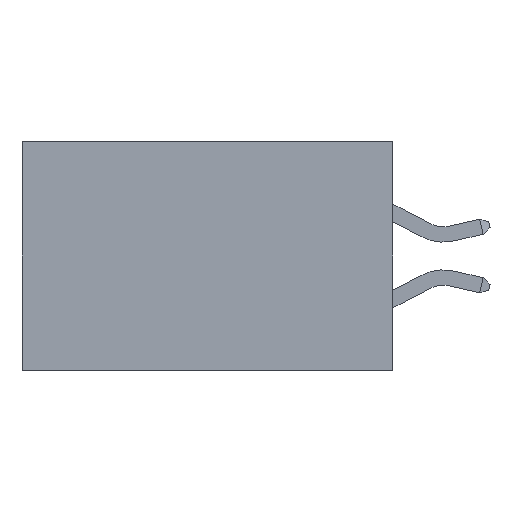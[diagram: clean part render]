
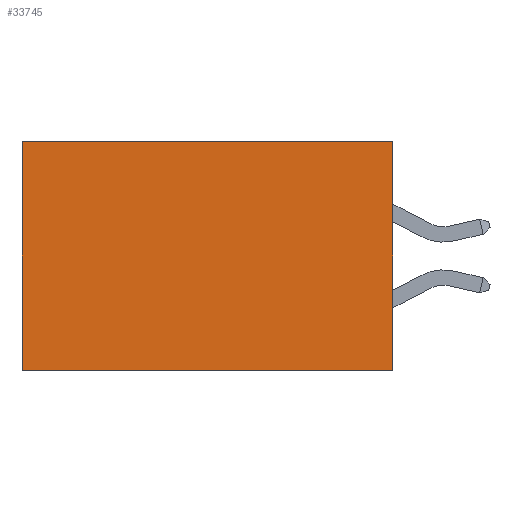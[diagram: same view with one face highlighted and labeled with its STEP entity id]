
A CAD part, left-side view. The second image highlights one B-rep face of the part: STEP entity #33745.
In plain terms, the highlighted planar face has unit normal (-1, 0, 0).
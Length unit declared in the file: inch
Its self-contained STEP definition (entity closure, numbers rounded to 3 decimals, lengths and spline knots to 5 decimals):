
#3464 = CARTESIAN_POINT ( 'NONE',  ( 0.2875, 0., 0. ) ) ;
#3906 = EDGE_CURVE ( 'NONE', #8949, #22092, #23940, .T. ) ;
#4215 = AXIS2_PLACEMENT_3D ( 'NONE', #3464, #6628, #9650 ) ;
#6011 = CARTESIAN_POINT ( 'NONE',  ( 0.2875, 0.6, 0. ) ) ;
#6628 = DIRECTION ( 'NONE',  ( 1., 0., 0. ) ) ;
#8949 = VERTEX_POINT ( 'NONE', #38374 ) ;
#9650 = DIRECTION ( 'NONE',  ( 0., 0., -1. ) ) ;
#9981 = ORIENTED_EDGE ( 'NONE', *, *, #10531, .F. ) ;
#10531 = EDGE_CURVE ( 'NONE', #20778, #22092, #31331, .T. ) ;
#10961 = LINE ( 'NONE', #13908, #26817 ) ;
#11271 = DIRECTION ( 'NONE',  ( 0., 1., 0. ) ) ;
#12602 = EDGE_CURVE ( 'NONE', #16168, #8949, #10961, .T. ) ;
#13908 = CARTESIAN_POINT ( 'NONE',  ( 0.2875, 0., 0. ) ) ;
#14796 = DIRECTION ( 'NONE',  ( 0., 0., -1. ) ) ;
#15211 = CARTESIAN_POINT ( 'NONE',  ( 0.2875, 0., -0.37 ) ) ;
#16168 = VERTEX_POINT ( 'NONE', #17316 ) ;
#17316 = CARTESIAN_POINT ( 'NONE',  ( 0.2875, 0., 0. ) ) ;
#17751 = EDGE_CURVE ( 'NONE', #16168, #20778, #32588, .T. ) ;
#18382 = CARTESIAN_POINT ( 'NONE',  ( 0.2875, 0., 0. ) ) ;
#20222 = ORIENTED_EDGE ( 'NONE', *, *, #17751, .F. ) ;
#20778 = VERTEX_POINT ( 'NONE', #15211 ) ;
#21093 = DIRECTION ( 'NONE',  ( 0., 0., -1. ) ) ;
#21530 = PLANE ( 'NONE',  #4215 ) ;
#21616 = VECTOR ( 'NONE', #14796, 39.37008 ) ;
#22092 = VERTEX_POINT ( 'NONE', #32736 ) ;
#23940 = LINE ( 'NONE', #6011, #21616 ) ;
#26817 = VECTOR ( 'NONE', #11271, 39.37008 ) ;
#27501 = FACE_OUTER_BOUND ( 'NONE', #28050, .T. ) ;
#28050 = EDGE_LOOP ( 'NONE', ( #33473, #9981, #20222, #31656 ) ) ;
#28995 = VECTOR ( 'NONE', #36642, 39.37008 ) ;
#30617 = CARTESIAN_POINT ( 'NONE',  ( 0.2875, 0., -0.37 ) ) ;
#30713 = VECTOR ( 'NONE', #21093, 39.37008 ) ;
#31331 = LINE ( 'NONE', #30617, #28995 ) ;
#31656 = ORIENTED_EDGE ( 'NONE', *, *, #12602, .T. ) ;
#32588 = LINE ( 'NONE', #18382, #30713 ) ;
#32736 = CARTESIAN_POINT ( 'NONE',  ( 0.2875, 0.6, -0.37 ) ) ;
#33473 = ORIENTED_EDGE ( 'NONE', *, *, #3906, .T. ) ;
#33745 = ADVANCED_FACE ( 'NONE', ( #27501 ), #21530, .F. ) ;
#36642 = DIRECTION ( 'NONE',  ( 0., 1., 0. ) ) ;
#38374 = CARTESIAN_POINT ( 'NONE',  ( 0.2875, 0.6, 0. ) ) ;
